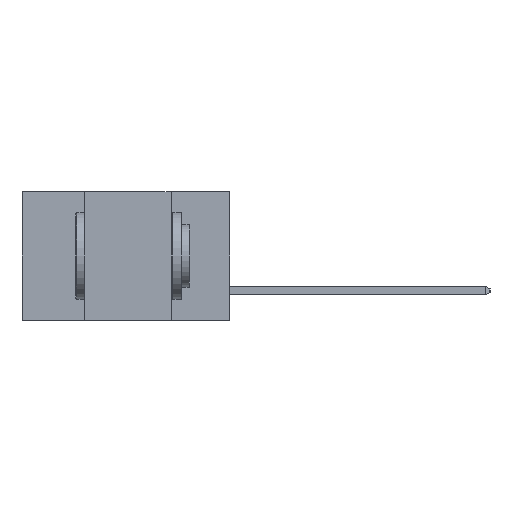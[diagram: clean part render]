
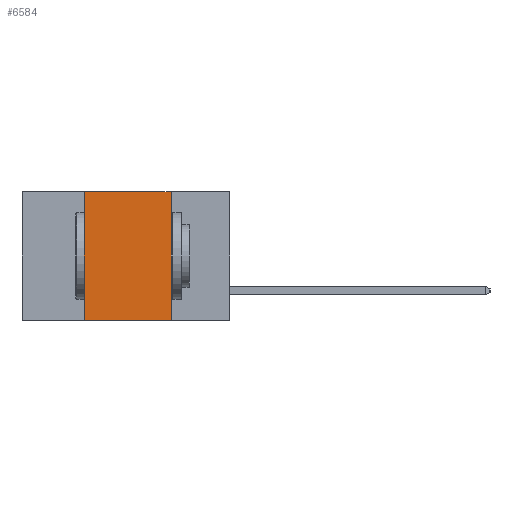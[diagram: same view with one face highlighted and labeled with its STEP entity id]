
A CAD part, left-side view. The second image highlights one B-rep face of the part: STEP entity #6584.
In plain terms, the highlighted planar face has unit normal (-1, 0, 0).
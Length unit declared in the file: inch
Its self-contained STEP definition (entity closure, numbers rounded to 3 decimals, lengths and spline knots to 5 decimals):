
#75 = LINE ( 'NONE', #23094, #4716 ) ;
#1041 = AXIS2_PLACEMENT_3D ( 'NONE', #21794, #21712, #21693 ) ;
#1538 = CARTESIAN_POINT ( 'NONE',  ( 0., 0.42, 0. ) ) ;
#2155 = ORIENTED_EDGE ( 'NONE', *, *, #6823, .T. ) ;
#2230 = CARTESIAN_POINT ( 'NONE',  ( 0., 0.17, -0.37 ) ) ;
#2375 = EDGE_CURVE ( 'NONE', #10873, #13861, #9521, .T. ) ;
#2578 = VECTOR ( 'NONE', #14738, 39.37008 ) ;
#2932 = CARTESIAN_POINT ( 'NONE',  ( 0., 0.42, 0. ) ) ;
#4506 = VECTOR ( 'NONE', #9508, 39.37008 ) ;
#4716 = VECTOR ( 'NONE', #15953, 39.37008 ) ;
#5669 = VECTOR ( 'NONE', #14743, 39.37008 ) ;
#6584 = ADVANCED_FACE ( 'NONE', ( #7163 ), #22264, .F. ) ;
#6823 = EDGE_CURVE ( 'NONE', #11765, #9087, #10637, .T. ) ;
#7089 = LINE ( 'NONE', #1538, #2578 ) ;
#7163 = FACE_OUTER_BOUND ( 'NONE', #14850, .T. ) ;
#9087 = VERTEX_POINT ( 'NONE', #2230 ) ;
#9302 = CARTESIAN_POINT ( 'NONE',  ( 0., 0.42, -0.37 ) ) ;
#9508 = DIRECTION ( 'NONE',  ( 0., -1., 0. ) ) ;
#9521 = LINE ( 'NONE', #11070, #4506 ) ;
#10637 = LINE ( 'NONE', #15380, #5669 ) ;
#10873 = VERTEX_POINT ( 'NONE', #2932 ) ;
#11013 = EDGE_CURVE ( 'NONE', #11765, #10873, #7089, .T. ) ;
#11070 = CARTESIAN_POINT ( 'NONE',  ( 0., 0.6, 0. ) ) ;
#11765 = VERTEX_POINT ( 'NONE', #9302 ) ;
#13861 = VERTEX_POINT ( 'NONE', #17577 ) ;
#14738 = DIRECTION ( 'NONE',  ( 0., 0., 1. ) ) ;
#14743 = DIRECTION ( 'NONE',  ( 0., -1., 0. ) ) ;
#14850 = EDGE_LOOP ( 'NONE', ( #17318, #22686, #15918, #2155 ) ) ;
#15380 = CARTESIAN_POINT ( 'NONE',  ( 0., 0.6, -0.37 ) ) ;
#15918 = ORIENTED_EDGE ( 'NONE', *, *, #11013, .F. ) ;
#15953 = DIRECTION ( 'NONE',  ( 0., 0., -1. ) ) ;
#17318 = ORIENTED_EDGE ( 'NONE', *, *, #23155, .F. ) ;
#17577 = CARTESIAN_POINT ( 'NONE',  ( 0., 0.17, 0. ) ) ;
#21693 = DIRECTION ( 'NONE',  ( 0., 0., -1. ) ) ;
#21712 = DIRECTION ( 'NONE',  ( 1., 0., 0. ) ) ;
#21794 = CARTESIAN_POINT ( 'NONE',  ( 0., 0.6, 0. ) ) ;
#22264 = PLANE ( 'NONE',  #1041 ) ;
#22686 = ORIENTED_EDGE ( 'NONE', *, *, #2375, .F. ) ;
#23094 = CARTESIAN_POINT ( 'NONE',  ( 0., 0.17, 0. ) ) ;
#23155 = EDGE_CURVE ( 'NONE', #13861, #9087, #75, .T. ) ;
